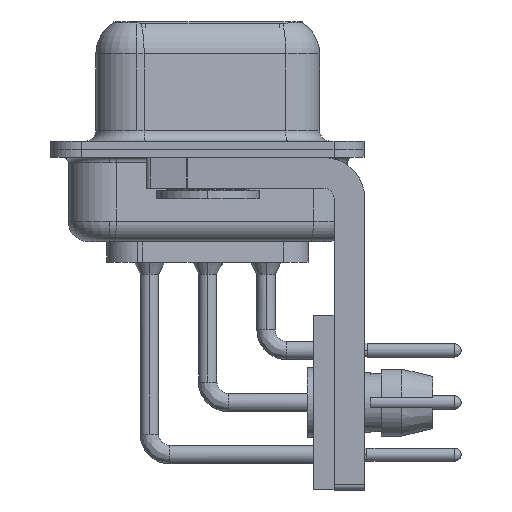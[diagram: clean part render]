
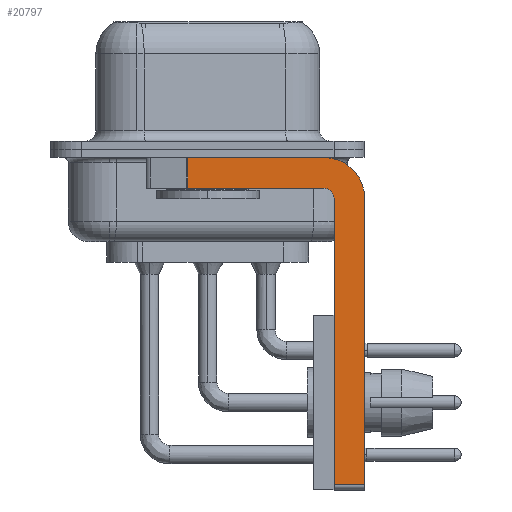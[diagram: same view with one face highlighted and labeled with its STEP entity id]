
A CAD part, left-side view. The second image highlights one B-rep face of the part: STEP entity #20797.
In plain terms, the highlighted planar face has unit normal (-1, 0, 0).
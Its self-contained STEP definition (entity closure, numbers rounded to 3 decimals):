
#307 = CARTESIAN_POINT ( 'NONE',  ( -2.9, -7.65, -16.35 ) ) ;
#1952 = VECTOR ( 'NONE', #17126, 1000. ) ;
#2213 = ORIENTED_EDGE ( 'NONE', *, *, #23142, .F. ) ;
#2705 = CARTESIAN_POINT ( 'NONE',  ( -2.9, 0.978, -1.9 ) ) ;
#2915 = LINE ( 'NONE', #20015, #1952 ) ;
#2996 = DIRECTION ( 'NONE',  ( 0., 0., -1. ) ) ;
#3345 = DIRECTION ( 'NONE',  ( 0., 0., 1. ) ) ;
#3479 = EDGE_CURVE ( 'NONE', #17411, #9518, #13752, .T. ) ;
#4857 = ORIENTED_EDGE ( 'NONE', *, *, #23565, .F. ) ;
#5133 = CARTESIAN_POINT ( 'NONE',  ( -2.9, -7.65, -2.4 ) ) ;
#5269 = DIRECTION ( 'NONE',  ( 0., 1., 0. ) ) ;
#5412 = CIRCLE ( 'NONE', #18436, 0.5 ) ;
#5449 = CARTESIAN_POINT ( 'NONE',  ( -2.9, 0.978, -0.4 ) ) ;
#6198 = EDGE_CURVE ( 'NONE', #36624, #29023, #8766, .T. ) ;
#6523 = CARTESIAN_POINT ( 'NONE',  ( -2.9, -5.65, -1.9 ) ) ;
#7055 = LINE ( 'NONE', #2705, #38589 ) ;
#7326 = DIRECTION ( 'NONE',  ( 0., 0., -1. ) ) ;
#8023 = CARTESIAN_POINT ( 'NONE',  ( -2.9, 0.978, -1.9 ) ) ;
#8766 = LINE ( 'NONE', #24605, #9754 ) ;
#9048 = ORIENTED_EDGE ( 'NONE', *, *, #33529, .F. ) ;
#9518 = VERTEX_POINT ( 'NONE', #8023 ) ;
#9754 = VECTOR ( 'NONE', #2996, 1000. ) ;
#10196 = CARTESIAN_POINT ( 'NONE',  ( -2.9, -6.15, -2.4 ) ) ;
#10330 = CARTESIAN_POINT ( 'NONE',  ( -2.9, -5.65, -2.4 ) ) ;
#12059 = DIRECTION ( 'NONE',  ( 1., 0., 0. ) ) ;
#12756 = VECTOR ( 'NONE', #5269, 1000. ) ;
#13072 = CARTESIAN_POINT ( 'NONE',  ( -2.9, -5.65, -0.4 ) ) ;
#13403 = ORIENTED_EDGE ( 'NONE', *, *, #3479, .F. ) ;
#13752 = LINE ( 'NONE', #6523, #12756 ) ;
#14533 = VECTOR ( 'NONE', #3345, 1000. ) ;
#15088 = DIRECTION ( 'NONE',  ( 0., 0., -1. ) ) ;
#16632 = DIRECTION ( 'NONE',  ( -1., 0., 0. ) ) ;
#17126 = DIRECTION ( 'NONE',  ( 0., -1., 0. ) ) ;
#17411 = VERTEX_POINT ( 'NONE', #25643 ) ;
#17919 = VERTEX_POINT ( 'NONE', #10196 ) ;
#18370 = VERTEX_POINT ( 'NONE', #5449 ) ;
#18436 = AXIS2_PLACEMENT_3D ( 'NONE', #34844, #16632, #37902 ) ;
#18573 = EDGE_CURVE ( 'NONE', #20543, #17919, #22589, .T. ) ;
#18578 = ORIENTED_EDGE ( 'NONE', *, *, #20024, .T. ) ;
#20015 = CARTESIAN_POINT ( 'NONE',  ( -2.9, 3., -0.4 ) ) ;
#20024 = EDGE_CURVE ( 'NONE', #18370, #9518, #7055, .T. ) ;
#20543 = VERTEX_POINT ( 'NONE', #27226 ) ;
#20797 = ADVANCED_FACE ( 'NONE', ( #31858 ), #22548, .F. ) ;
#20886 = VECTOR ( 'NONE', #26687, 1000. ) ;
#22548 = PLANE ( 'NONE',  #34140 ) ;
#22589 = LINE ( 'NONE', #33898, #14533 ) ;
#23142 = EDGE_CURVE ( 'NONE', #30395, #36624, #37406, .T. ) ;
#23565 = EDGE_CURVE ( 'NONE', #18370, #30395, #2915, .T. ) ;
#23650 = CARTESIAN_POINT ( 'NONE',  ( -2.9, -5.65, -16.35 ) ) ;
#24605 = CARTESIAN_POINT ( 'NONE',  ( -2.9, -7.65, -2.4 ) ) ;
#25600 = DIRECTION ( 'NONE',  ( 1., 0., 0. ) ) ;
#25643 = CARTESIAN_POINT ( 'NONE',  ( -2.9, -5.65, -1.9 ) ) ;
#25861 = ORIENTED_EDGE ( 'NONE', *, *, #31048, .T. ) ;
#26687 = DIRECTION ( 'NONE',  ( 0., -1., 0. ) ) ;
#27226 = CARTESIAN_POINT ( 'NONE',  ( -2.9, -6.15, -16.35 ) ) ;
#29023 = VERTEX_POINT ( 'NONE', #307 ) ;
#30317 = CARTESIAN_POINT ( 'NONE',  ( -2.9, -5.65, -2.4 ) ) ;
#30395 = VERTEX_POINT ( 'NONE', #13072 ) ;
#30656 = AXIS2_PLACEMENT_3D ( 'NONE', #30317, #12059, #33352 ) ;
#30715 = EDGE_LOOP ( 'NONE', ( #4857, #18578, #13403, #9048, #35024, #25861, #31514, #2213 ) ) ;
#31048 = EDGE_CURVE ( 'NONE', #20543, #29023, #37096, .T. ) ;
#31514 = ORIENTED_EDGE ( 'NONE', *, *, #6198, .F. ) ;
#31858 = FACE_OUTER_BOUND ( 'NONE', #30715, .T. ) ;
#33352 = DIRECTION ( 'NONE',  ( 0., 0., -1. ) ) ;
#33529 = EDGE_CURVE ( 'NONE', #17919, #17411, #5412, .T. ) ;
#33898 = CARTESIAN_POINT ( 'NONE',  ( -2.9, -6.15, -16.6 ) ) ;
#34140 = AXIS2_PLACEMENT_3D ( 'NONE', #10330, #25600, #7326 ) ;
#34844 = CARTESIAN_POINT ( 'NONE',  ( -2.9, -5.65, -2.4 ) ) ;
#35024 = ORIENTED_EDGE ( 'NONE', *, *, #18573, .F. ) ;
#36624 = VERTEX_POINT ( 'NONE', #5133 ) ;
#37096 = LINE ( 'NONE', #23650, #20886 ) ;
#37406 = CIRCLE ( 'NONE', #30656, 2. ) ;
#37902 = DIRECTION ( 'NONE',  ( 0., 0., 1. ) ) ;
#38589 = VECTOR ( 'NONE', #15088, 1000. ) ;
